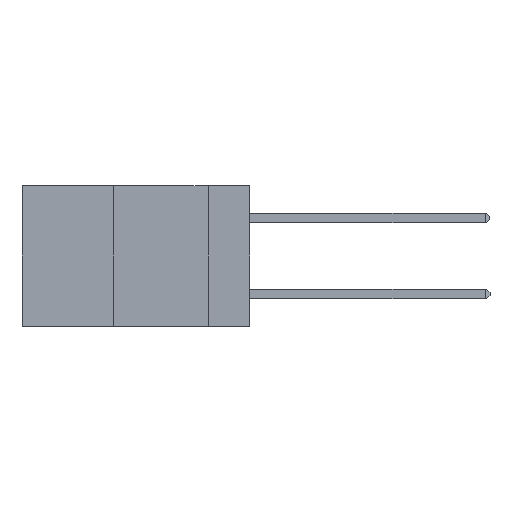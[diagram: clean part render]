
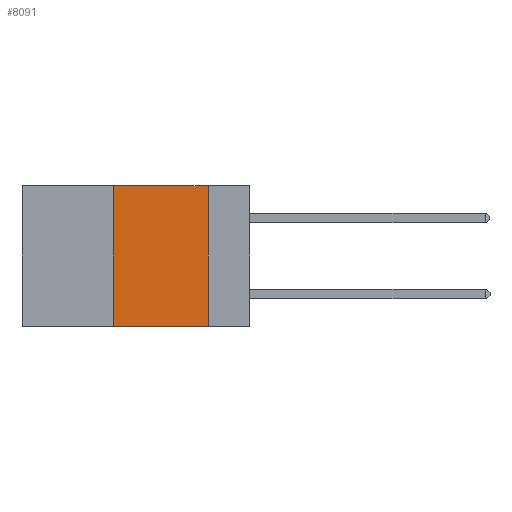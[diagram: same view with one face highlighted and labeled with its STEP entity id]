
A CAD part, left-side view. The second image highlights one B-rep face of the part: STEP entity #8091.
In plain terms, the highlighted planar face has unit normal (-1, 0, 0).
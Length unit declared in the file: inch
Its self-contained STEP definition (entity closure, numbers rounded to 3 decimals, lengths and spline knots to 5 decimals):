
#1189 = CARTESIAN_POINT ( 'NONE',  ( 0., 0.6, 0. ) ) ;
#1490 = ORIENTED_EDGE ( 'NONE', *, *, #7922, .F. ) ;
#2417 = DIRECTION ( 'NONE',  ( 0., 0., -1. ) ) ;
#3092 = VERTEX_POINT ( 'NONE', #10441 ) ;
#3159 = VECTOR ( 'NONE', #8461, 39.37008 ) ;
#3365 = FACE_OUTER_BOUND ( 'NONE', #7762, .T. ) ;
#4162 = VERTEX_POINT ( 'NONE', #8894 ) ;
#5341 = CARTESIAN_POINT ( 'NONE',  ( 0., 0.11, 0. ) ) ;
#5717 = CARTESIAN_POINT ( 'NONE',  ( 0., 0.36, 0. ) ) ;
#6497 = LINE ( 'NONE', #8646, #6960 ) ;
#6958 = LINE ( 'NONE', #16596, #3159 ) ;
#6960 = VECTOR ( 'NONE', #18123, 39.37008 ) ;
#7762 = EDGE_LOOP ( 'NONE', ( #1490, #16396, #14949, #8539 ) ) ;
#7922 = EDGE_CURVE ( 'NONE', #3092, #10143, #16129, .T. ) ;
#8091 = ADVANCED_FACE ( 'NONE', ( #3365 ), #15283, .F. ) ;
#8117 = VERTEX_POINT ( 'NONE', #5717 ) ;
#8461 = DIRECTION ( 'NONE',  ( 0., -1., 0. ) ) ;
#8487 = DIRECTION ( 'NONE',  ( 0., 0., -1. ) ) ;
#8491 = CARTESIAN_POINT ( 'NONE',  ( 0., 0.11, -0.37 ) ) ;
#8539 = ORIENTED_EDGE ( 'NONE', *, *, #15257, .T. ) ;
#8646 = CARTESIAN_POINT ( 'NONE',  ( 0., 0.36, 0. ) ) ;
#8870 = EDGE_CURVE ( 'NONE', #4162, #8117, #6497, .T. ) ;
#8894 = CARTESIAN_POINT ( 'NONE',  ( 0., 0.36, -0.37 ) ) ;
#9425 = LINE ( 'NONE', #11769, #13129 ) ;
#9947 = AXIS2_PLACEMENT_3D ( 'NONE', #1189, #16624, #8487 ) ;
#10143 = VERTEX_POINT ( 'NONE', #8491 ) ;
#10441 = CARTESIAN_POINT ( 'NONE',  ( 0., 0.11, 0. ) ) ;
#11769 = CARTESIAN_POINT ( 'NONE',  ( 0., 0.6, 0. ) ) ;
#13116 = DIRECTION ( 'NONE',  ( 0., -1., 0. ) ) ;
#13125 = EDGE_CURVE ( 'NONE', #8117, #3092, #9425, .T. ) ;
#13129 = VECTOR ( 'NONE', #13116, 39.37008 ) ;
#14949 = ORIENTED_EDGE ( 'NONE', *, *, #8870, .F. ) ;
#15257 = EDGE_CURVE ( 'NONE', #4162, #10143, #6958, .T. ) ;
#15283 = PLANE ( 'NONE',  #9947 ) ;
#15723 = VECTOR ( 'NONE', #2417, 39.37008 ) ;
#16129 = LINE ( 'NONE', #5341, #15723 ) ;
#16396 = ORIENTED_EDGE ( 'NONE', *, *, #13125, .F. ) ;
#16596 = CARTESIAN_POINT ( 'NONE',  ( 0., 0.6, -0.37 ) ) ;
#16624 = DIRECTION ( 'NONE',  ( 1., 0., 0. ) ) ;
#18123 = DIRECTION ( 'NONE',  ( 0., 0., 1. ) ) ;
